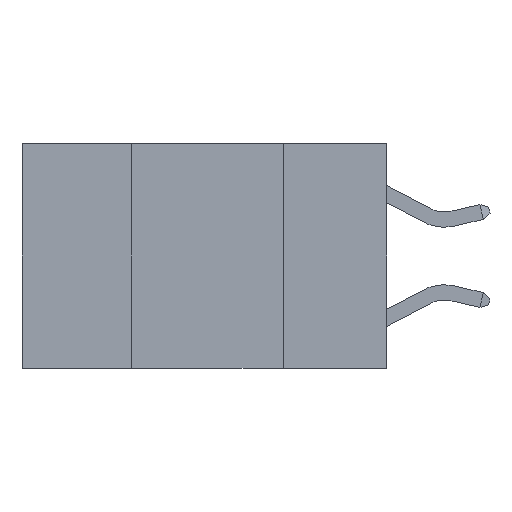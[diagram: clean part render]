
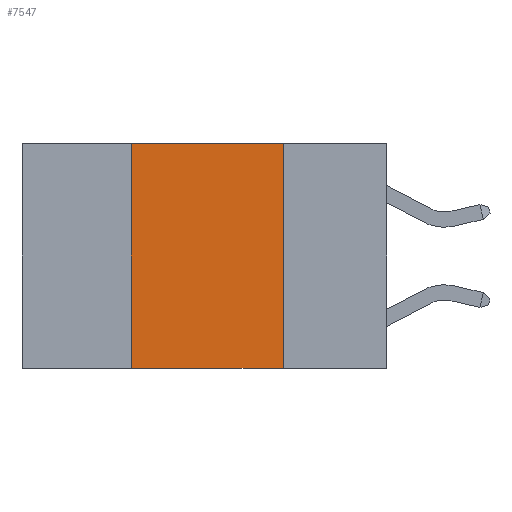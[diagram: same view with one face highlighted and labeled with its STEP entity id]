
A CAD part, left-side view. The second image highlights one B-rep face of the part: STEP entity #7547.
In plain terms, the highlighted planar face has unit normal (-1, 0, 0).
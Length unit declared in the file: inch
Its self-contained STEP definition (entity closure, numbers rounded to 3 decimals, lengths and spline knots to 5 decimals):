
#836 = LINE ( 'NONE', #2448, #6269 ) ;
#1215 = ORIENTED_EDGE ( 'NONE', *, *, #3655, .F. ) ;
#1363 = DIRECTION ( 'NONE',  ( 0., -1., 0. ) ) ;
#1489 = ORIENTED_EDGE ( 'NONE', *, *, #5420, .F. ) ;
#1500 = VECTOR ( 'NONE', #2550, 39.37008 ) ;
#1631 = CARTESIAN_POINT ( 'NONE',  ( 0., 0.42, 0. ) ) ;
#2069 = CARTESIAN_POINT ( 'NONE',  ( 0., 0.6, -0.37 ) ) ;
#2124 = VERTEX_POINT ( 'NONE', #8071 ) ;
#2376 = CARTESIAN_POINT ( 'NONE',  ( 0., 0.6, 0. ) ) ;
#2414 = DIRECTION ( 'NONE',  ( 0., 0., 1. ) ) ;
#2448 = CARTESIAN_POINT ( 'NONE',  ( 0., 0.42, 0. ) ) ;
#2550 = DIRECTION ( 'NONE',  ( 0., 0., -1. ) ) ;
#2713 = EDGE_LOOP ( 'NONE', ( #5040, #1215, #1489, #5741 ) ) ;
#2823 = DIRECTION ( 'NONE',  ( 0., -1., 0. ) ) ;
#2855 = VECTOR ( 'NONE', #1363, 39.37008 ) ;
#3196 = LINE ( 'NONE', #8801, #1500 ) ;
#3292 = CARTESIAN_POINT ( 'NONE',  ( 0., 0.17, -0.37 ) ) ;
#3552 = VECTOR ( 'NONE', #2823, 39.37008 ) ;
#3601 = CARTESIAN_POINT ( 'NONE',  ( 0., 0.42, -0.37 ) ) ;
#3655 = EDGE_CURVE ( 'NONE', #8612, #2124, #7230, .T. ) ;
#3796 = DIRECTION ( 'NONE',  ( 0., 0., -1. ) ) ;
#4168 = VERTEX_POINT ( 'NONE', #3292 ) ;
#4552 = VERTEX_POINT ( 'NONE', #3601 ) ;
#4690 = LINE ( 'NONE', #2069, #2855 ) ;
#4883 = CARTESIAN_POINT ( 'NONE',  ( 0., 0.6, 0. ) ) ;
#5040 = ORIENTED_EDGE ( 'NONE', *, *, #7042, .F. ) ;
#5420 = EDGE_CURVE ( 'NONE', #4552, #8612, #836, .T. ) ;
#5741 = ORIENTED_EDGE ( 'NONE', *, *, #7719, .T. ) ;
#6192 = AXIS2_PLACEMENT_3D ( 'NONE', #2376, #7929, #3796 ) ;
#6219 = FACE_OUTER_BOUND ( 'NONE', #2713, .T. ) ;
#6269 = VECTOR ( 'NONE', #2414, 39.37008 ) ;
#6549 = PLANE ( 'NONE',  #6192 ) ;
#7042 = EDGE_CURVE ( 'NONE', #2124, #4168, #3196, .T. ) ;
#7230 = LINE ( 'NONE', #4883, #3552 ) ;
#7547 = ADVANCED_FACE ( 'NONE', ( #6219 ), #6549, .F. ) ;
#7719 = EDGE_CURVE ( 'NONE', #4552, #4168, #4690, .T. ) ;
#7929 = DIRECTION ( 'NONE',  ( 1., 0., 0. ) ) ;
#8071 = CARTESIAN_POINT ( 'NONE',  ( 0., 0.17, 0. ) ) ;
#8612 = VERTEX_POINT ( 'NONE', #1631 ) ;
#8801 = CARTESIAN_POINT ( 'NONE',  ( 0., 0.17, 0. ) ) ;
